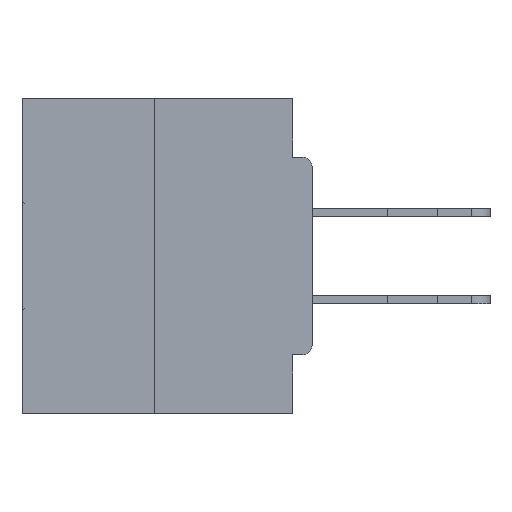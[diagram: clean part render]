
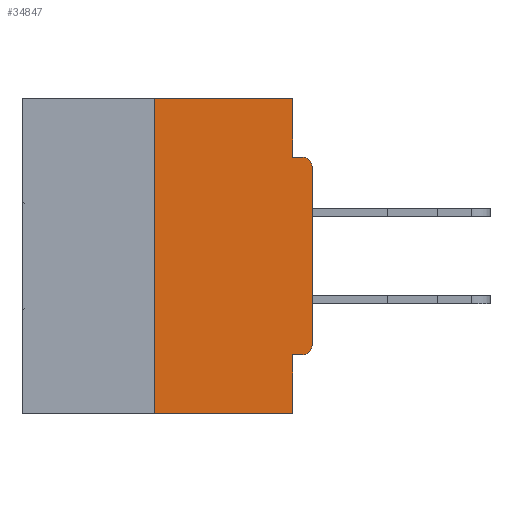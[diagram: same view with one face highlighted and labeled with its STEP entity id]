
A CAD part, left-side view. The second image highlights one B-rep face of the part: STEP entity #34847.
In plain terms, the highlighted planar face has unit normal (-1, 0, 0).
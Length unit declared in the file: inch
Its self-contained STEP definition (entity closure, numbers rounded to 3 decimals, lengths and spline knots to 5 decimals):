
#940 = DIRECTION ( 'NONE',  ( -1., 0., 0. ) ) ;
#1149 = ORIENTED_EDGE ( 'NONE', *, *, #23240, .F. ) ;
#2451 = EDGE_CURVE ( 'NONE', #18336, #37773, #38646, .T. ) ;
#2798 = LINE ( 'NONE', #38896, #17967 ) ;
#4023 = ORIENTED_EDGE ( 'NONE', *, *, #8729, .F. ) ;
#4429 = CARTESIAN_POINT ( 'NONE',  ( 0., 0., -0.0935 ) ) ;
#4845 = DIRECTION ( 'NONE',  ( 0., 0., -1. ) ) ;
#5108 = ORIENTED_EDGE ( 'NONE', *, *, #22748, .T. ) ;
#5209 = VECTOR ( 'NONE', #31702, 39.37008 ) ;
#5808 = FACE_OUTER_BOUND ( 'NONE', #39212, .T. ) ;
#5903 = ORIENTED_EDGE ( 'NONE', *, *, #6501, .F. ) ;
#6305 = CARTESIAN_POINT ( 'NONE',  ( 0., 0., -0.3915 ) ) ;
#6501 = EDGE_CURVE ( 'NONE', #27470, #32365, #24198, .T. ) ;
#6555 = VERTEX_POINT ( 'NONE', #8202 ) ;
#8202 = CARTESIAN_POINT ( 'NONE',  ( 0., 0.015, -0.0935 ) ) ;
#8551 = DIRECTION ( 'NONE',  ( -1., 0., 0. ) ) ;
#8729 = EDGE_CURVE ( 'NONE', #32365, #6555, #21214, .T. ) ;
#9193 = CARTESIAN_POINT ( 'NONE',  ( 0., 0.25, 0. ) ) ;
#9882 = EDGE_CURVE ( 'NONE', #40071, #26665, #40825, .T. ) ;
#10071 = DIRECTION ( 'NONE',  ( 0., -1., 0. ) ) ;
#10139 = DIRECTION ( 'NONE',  ( 0., 0., -1. ) ) ;
#11123 = VECTOR ( 'NONE', #27010, 39.37008 ) ;
#11934 = DIRECTION ( 'NONE',  ( 0., 0., -1. ) ) ;
#12213 = CIRCLE ( 'NONE', #26248, 0.015 ) ;
#12470 = VECTOR ( 'NONE', #40225, 39.37008 ) ;
#13806 = LINE ( 'NONE', #9193, #5209 ) ;
#13817 = PLANE ( 'NONE',  #38594 ) ;
#14039 = VERTEX_POINT ( 'NONE', #14648 ) ;
#14097 = DIRECTION ( 'NONE',  ( 0., 0., -1. ) ) ;
#14122 = VECTOR ( 'NONE', #37058, 39.37008 ) ;
#14302 = CARTESIAN_POINT ( 'NONE',  ( 0., 0.031, 0. ) ) ;
#14365 = CARTESIAN_POINT ( 'NONE',  ( 0., 0., -0.1085 ) ) ;
#14648 = CARTESIAN_POINT ( 'NONE',  ( 0., 0.25, 0. ) ) ;
#16288 = CARTESIAN_POINT ( 'NONE',  ( 0., 0.031, -0.4065 ) ) ;
#16473 = VERTEX_POINT ( 'NONE', #14365 ) ;
#16576 = DIRECTION ( 'NONE',  ( 0., -1., 0. ) ) ;
#17639 = CARTESIAN_POINT ( 'NONE',  ( 0., 0., 0. ) ) ;
#17759 = VECTOR ( 'NONE', #16576, 39.37008 ) ;
#17967 = VECTOR ( 'NONE', #10071, 39.37008 ) ;
#18336 = VERTEX_POINT ( 'NONE', #16288 ) ;
#21017 = CARTESIAN_POINT ( 'NONE',  ( 0., 0.015, -0.4065 ) ) ;
#21133 = CARTESIAN_POINT ( 'NONE',  ( 0., 0.031, 0. ) ) ;
#21214 = LINE ( 'NONE', #4429, #11123 ) ;
#21681 = EDGE_CURVE ( 'NONE', #40071, #18336, #33041, .T. ) ;
#21773 = ORIENTED_EDGE ( 'NONE', *, *, #2451, .F. ) ;
#22437 = ORIENTED_EDGE ( 'NONE', *, *, #33718, .T. ) ;
#22542 = CARTESIAN_POINT ( 'NONE',  ( 0., 0.015, -0.3915 ) ) ;
#22748 = EDGE_CURVE ( 'NONE', #16473, #6555, #12213, .T. ) ;
#22880 = VECTOR ( 'NONE', #40752, 39.37008 ) ;
#23240 = EDGE_CURVE ( 'NONE', #14039, #27470, #27374, .T. ) ;
#24198 = LINE ( 'NONE', #14302, #14122 ) ;
#24205 = CARTESIAN_POINT ( 'NONE',  ( 0., 0.031, -0.0935 ) ) ;
#24751 = CARTESIAN_POINT ( 'NONE',  ( 0., 0.25, -0.5 ) ) ;
#24768 = ORIENTED_EDGE ( 'NONE', *, *, #9882, .T. ) ;
#26248 = AXIS2_PLACEMENT_3D ( 'NONE', #27501, #940, #10139 ) ;
#26665 = VERTEX_POINT ( 'NONE', #6305 ) ;
#26819 = CARTESIAN_POINT ( 'NONE',  ( 0., 0.46, 0. ) ) ;
#27010 = DIRECTION ( 'NONE',  ( 0., -1., 0. ) ) ;
#27374 = LINE ( 'NONE', #32720, #17759 ) ;
#27470 = VERTEX_POINT ( 'NONE', #21133 ) ;
#27501 = CARTESIAN_POINT ( 'NONE',  ( 0., 0.015, -0.1085 ) ) ;
#27673 = ORIENTED_EDGE ( 'NONE', *, *, #38947, .F. ) ;
#31702 = DIRECTION ( 'NONE',  ( 0., 0., 1. ) ) ;
#32215 = LINE ( 'NONE', #17639, #12470 ) ;
#32365 = VERTEX_POINT ( 'NONE', #24205 ) ;
#32482 = ORIENTED_EDGE ( 'NONE', *, *, #21681, .F. ) ;
#32585 = VERTEX_POINT ( 'NONE', #24751 ) ;
#32720 = CARTESIAN_POINT ( 'NONE',  ( 0., 0.46, 0. ) ) ;
#32924 = ORIENTED_EDGE ( 'NONE', *, *, #34372, .T. ) ;
#33041 = LINE ( 'NONE', #37367, #22880 ) ;
#33718 = EDGE_CURVE ( 'NONE', #26665, #16473, #32215, .T. ) ;
#34277 = CARTESIAN_POINT ( 'NONE',  ( 0., 0.031, -0.5 ) ) ;
#34372 = EDGE_CURVE ( 'NONE', #32585, #37773, #2798, .T. ) ;
#34847 = ADVANCED_FACE ( 'NONE', ( #5808 ), #13817, .F. ) ;
#35671 = VECTOR ( 'NONE', #4845, 39.37008 ) ;
#37058 = DIRECTION ( 'NONE',  ( 0., 0., -1. ) ) ;
#37367 = CARTESIAN_POINT ( 'NONE',  ( 0., 0., -0.4065 ) ) ;
#37773 = VERTEX_POINT ( 'NONE', #37826 ) ;
#37826 = CARTESIAN_POINT ( 'NONE',  ( 0., 0.031, -0.5 ) ) ;
#38594 = AXIS2_PLACEMENT_3D ( 'NONE', #26819, #40075, #14097 ) ;
#38646 = LINE ( 'NONE', #34277, #35671 ) ;
#38896 = CARTESIAN_POINT ( 'NONE',  ( 0., 0.46, -0.5 ) ) ;
#38947 = EDGE_CURVE ( 'NONE', #32585, #14039, #13806, .T. ) ;
#39212 = EDGE_LOOP ( 'NONE', ( #1149, #27673, #32924, #21773, #32482, #24768, #22437, #5108, #4023, #5903 ) ) ;
#40071 = VERTEX_POINT ( 'NONE', #21017 ) ;
#40075 = DIRECTION ( 'NONE',  ( 1., 0., 0. ) ) ;
#40225 = DIRECTION ( 'NONE',  ( 0., 0., 1. ) ) ;
#40752 = DIRECTION ( 'NONE',  ( 0., 1., 0. ) ) ;
#40790 = AXIS2_PLACEMENT_3D ( 'NONE', #22542, #8551, #11934 ) ;
#40825 = CIRCLE ( 'NONE', #40790, 0.015 ) ;
